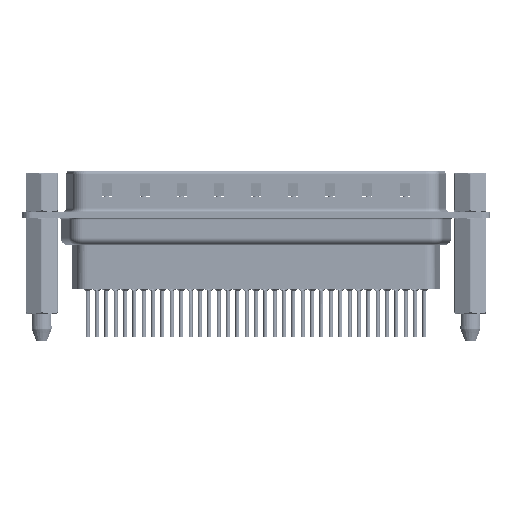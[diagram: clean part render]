
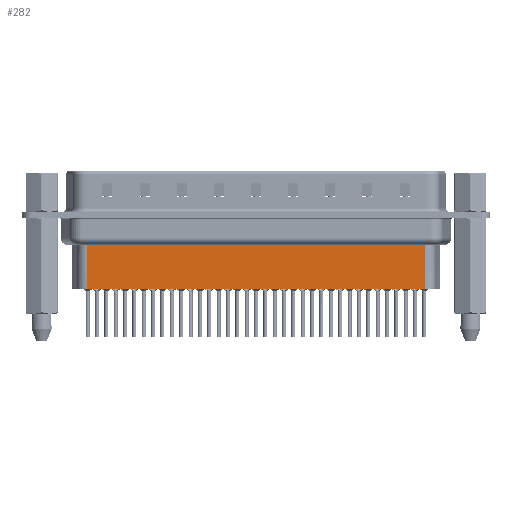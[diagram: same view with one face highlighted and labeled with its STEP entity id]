
A CAD part, front view. The second image highlights one B-rep face of the part: STEP entity #282.
In plain terms, the highlighted planar face has unit normal (0, -1, 0).
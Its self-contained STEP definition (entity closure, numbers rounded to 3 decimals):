
#90 = LINE ( 'NONE', #31176, #31699 ) ;
#282 = ADVANCED_FACE ( 'NONE', ( #13087 ), #26761, .T. ) ;
#1463 = VERTEX_POINT ( 'NONE', #5598 ) ;
#3130 = LINE ( 'NONE', #17201, #20122 ) ;
#3753 = LINE ( 'NONE', #7105, #21049 ) ;
#5354 = EDGE_CURVE ( 'NONE', #13082, #13763, #3753, .T. ) ;
#5598 = CARTESIAN_POINT ( 'NONE',  ( 6.706, -3.5, -10.95 ) ) ;
#6854 = VERTEX_POINT ( 'NONE', #19667 ) ;
#7105 = CARTESIAN_POINT ( 'NONE',  ( 56.794, -3.5, -3.1 ) ) ;
#8697 = DIRECTION ( 'NONE',  ( -1., 0., 0. ) ) ;
#9539 = DIRECTION ( 'NONE',  ( 1., 0., 0. ) ) ;
#11622 = ORIENTED_EDGE ( 'NONE', *, *, #5354, .F. ) ;
#12296 = VECTOR ( 'NONE', #25803, 1000. ) ;
#13082 = VERTEX_POINT ( 'NONE', #27628 ) ;
#13087 = FACE_OUTER_BOUND ( 'NONE', #30733, .T. ) ;
#13763 = VERTEX_POINT ( 'NONE', #32020 ) ;
#14387 = EDGE_CURVE ( 'NONE', #13763, #1463, #90, .T. ) ;
#14929 = LINE ( 'NONE', #20545, #12296 ) ;
#14932 = DIRECTION ( 'NONE',  ( 0., 0., -1. ) ) ;
#15525 = CARTESIAN_POINT ( 'NONE',  ( 6.706, -3.5, -3.1 ) ) ;
#17201 = CARTESIAN_POINT ( 'NONE',  ( 6.706, -3.5, -3.1 ) ) ;
#19667 = CARTESIAN_POINT ( 'NONE',  ( 6.706, -3.5, -4.097 ) ) ;
#20122 = VECTOR ( 'NONE', #14932, 1000. ) ;
#20545 = CARTESIAN_POINT ( 'NONE',  ( 6.459, -3.5, -4.097 ) ) ;
#21049 = VECTOR ( 'NONE', #34995, 1000. ) ;
#24819 = ORIENTED_EDGE ( 'NONE', *, *, #32083, .T. ) ;
#25154 = ORIENTED_EDGE ( 'NONE', *, *, #33616, .T. ) ;
#25622 = ORIENTED_EDGE ( 'NONE', *, *, #14387, .F. ) ;
#25803 = DIRECTION ( 'NONE',  ( -1., 0., 0. ) ) ;
#26761 = PLANE ( 'NONE',  #31946 ) ;
#27628 = CARTESIAN_POINT ( 'NONE',  ( 56.794, -3.5, -4.097 ) ) ;
#30309 = DIRECTION ( 'NONE',  ( 0., -1., 0. ) ) ;
#30733 = EDGE_LOOP ( 'NONE', ( #11622, #24819, #25154, #25622 ) ) ;
#31176 = CARTESIAN_POINT ( 'NONE',  ( 6.706, -3.5, -10.95 ) ) ;
#31699 = VECTOR ( 'NONE', #8697, 1000. ) ;
#31946 = AXIS2_PLACEMENT_3D ( 'NONE', #15525, #30309, #9539 ) ;
#32020 = CARTESIAN_POINT ( 'NONE',  ( 56.794, -3.5, -10.95 ) ) ;
#32083 = EDGE_CURVE ( 'NONE', #13082, #6854, #14929, .T. ) ;
#33616 = EDGE_CURVE ( 'NONE', #6854, #1463, #3130, .T. ) ;
#34995 = DIRECTION ( 'NONE',  ( 0., 0., -1. ) ) ;
